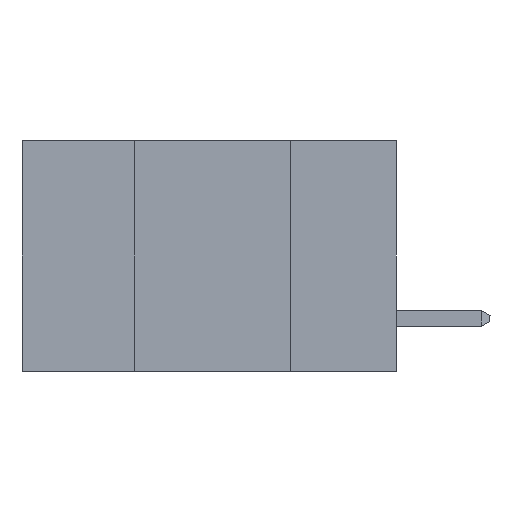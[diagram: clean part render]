
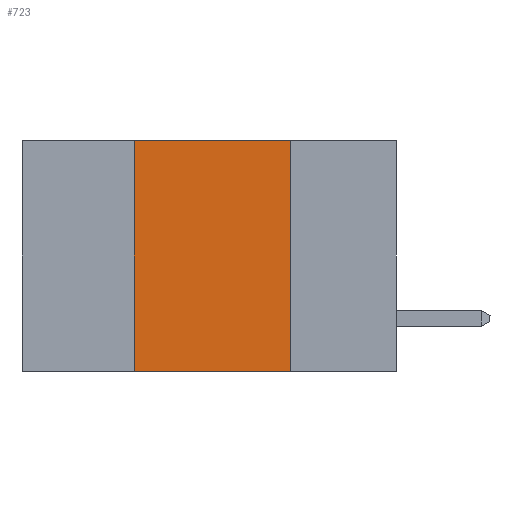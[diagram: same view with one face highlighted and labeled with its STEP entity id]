
A CAD part, left-side view. The second image highlights one B-rep face of the part: STEP entity #723.
In plain terms, the highlighted planar face has unit normal (-1, 0, 0).
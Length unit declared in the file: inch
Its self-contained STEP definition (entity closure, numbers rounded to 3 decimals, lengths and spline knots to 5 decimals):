
#130 = EDGE_CURVE ( 'NONE', #437, #595, #1336, .T. ) ;
#437 = VERTEX_POINT ( 'NONE', #5697 ) ;
#563 = DIRECTION ( 'NONE',  ( 0., -1., 0. ) ) ;
#595 = VERTEX_POINT ( 'NONE', #4616 ) ;
#723 = ADVANCED_FACE ( 'NONE', ( #3517 ), #4965, .F. ) ;
#753 = DIRECTION ( 'NONE',  ( 0., 0., 1. ) ) ;
#1336 = LINE ( 'NONE', #9716, #6684 ) ;
#2623 = VERTEX_POINT ( 'NONE', #8493 ) ;
#2963 = EDGE_CURVE ( 'NONE', #9282, #2623, #6068, .T. ) ;
#3260 = VECTOR ( 'NONE', #753, 39.37008 ) ;
#3324 = ORIENTED_EDGE ( 'NONE', *, *, #5646, .F. ) ;
#3517 = FACE_OUTER_BOUND ( 'NONE', #4578, .T. ) ;
#3802 = VECTOR ( 'NONE', #563, 39.37008 ) ;
#4202 = CARTESIAN_POINT ( 'NONE',  ( 0., 0.6, 0. ) ) ;
#4348 = LINE ( 'NONE', #9812, #8313 ) ;
#4528 = DIRECTION ( 'NONE',  ( 0., -1., 0. ) ) ;
#4571 = CARTESIAN_POINT ( 'NONE',  ( 0., 0.42, -0.37 ) ) ;
#4578 = EDGE_LOOP ( 'NONE', ( #9203, #3324, #7034, #7729 ) ) ;
#4616 = CARTESIAN_POINT ( 'NONE',  ( 0., 0.17, -0.37 ) ) ;
#4965 = PLANE ( 'NONE',  #8939 ) ;
#5431 = DIRECTION ( 'NONE',  ( 0., 0., -1. ) ) ;
#5606 = DIRECTION ( 'NONE',  ( 1., 0., 0. ) ) ;
#5646 = EDGE_CURVE ( 'NONE', #2623, #437, #6670, .T. ) ;
#5697 = CARTESIAN_POINT ( 'NONE',  ( 0., 0.17, 0. ) ) ;
#6068 = LINE ( 'NONE', #4571, #3260 ) ;
#6670 = LINE ( 'NONE', #7426, #3802 ) ;
#6684 = VECTOR ( 'NONE', #5431, 39.37008 ) ;
#7034 = ORIENTED_EDGE ( 'NONE', *, *, #2963, .F. ) ;
#7426 = CARTESIAN_POINT ( 'NONE',  ( 0., 0.6, 0. ) ) ;
#7729 = ORIENTED_EDGE ( 'NONE', *, *, #9387, .T. ) ;
#7925 = CARTESIAN_POINT ( 'NONE',  ( 0., 0.42, -0.37 ) ) ;
#8313 = VECTOR ( 'NONE', #4528, 39.37008 ) ;
#8493 = CARTESIAN_POINT ( 'NONE',  ( 0., 0.42, 0. ) ) ;
#8939 = AXIS2_PLACEMENT_3D ( 'NONE', #4202, #5606, #9579 ) ;
#9203 = ORIENTED_EDGE ( 'NONE', *, *, #130, .F. ) ;
#9282 = VERTEX_POINT ( 'NONE', #7925 ) ;
#9387 = EDGE_CURVE ( 'NONE', #9282, #595, #4348, .T. ) ;
#9579 = DIRECTION ( 'NONE',  ( 0., 0., -1. ) ) ;
#9716 = CARTESIAN_POINT ( 'NONE',  ( 0., 0.17, -0.37 ) ) ;
#9812 = CARTESIAN_POINT ( 'NONE',  ( 0., 0.6, -0.37 ) ) ;
